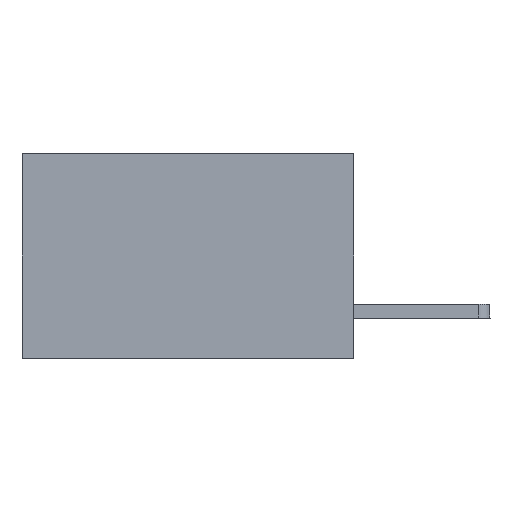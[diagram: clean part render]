
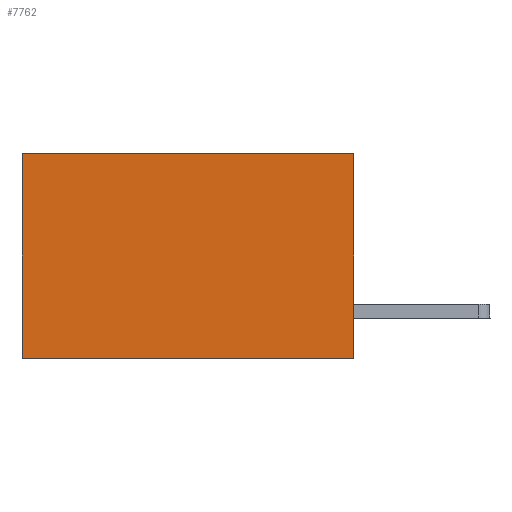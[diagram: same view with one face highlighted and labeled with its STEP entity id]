
A CAD part, left-side view. The second image highlights one B-rep face of the part: STEP entity #7762.
In plain terms, the highlighted planar face has unit normal (-1, 0, 0).
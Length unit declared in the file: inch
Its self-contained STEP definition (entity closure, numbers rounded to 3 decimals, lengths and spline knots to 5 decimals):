
#231 = VERTEX_POINT ( 'NONE', #5318 ) ;
#266 = CARTESIAN_POINT ( 'NONE',  ( 0.2875, 0.6, 0. ) ) ;
#314 = DIRECTION ( 'NONE',  ( 0., 0., -1. ) ) ;
#637 = ORIENTED_EDGE ( 'NONE', *, *, #11480, .T. ) ;
#988 = CARTESIAN_POINT ( 'NONE',  ( 0.2875, 0., 0. ) ) ;
#1458 = CARTESIAN_POINT ( 'NONE',  ( 0.2875, 0., 0. ) ) ;
#1547 = FACE_OUTER_BOUND ( 'NONE', #9340, .T. ) ;
#2187 = LINE ( 'NONE', #3910, #12727 ) ;
#2252 = CARTESIAN_POINT ( 'NONE',  ( 0.2875, 0., -0.37 ) ) ;
#2269 = ORIENTED_EDGE ( 'NONE', *, *, #9729, .T. ) ;
#2368 = DIRECTION ( 'NONE',  ( 0., 1., 0. ) ) ;
#3910 = CARTESIAN_POINT ( 'NONE',  ( 0.2875, 0., 0. ) ) ;
#3998 = VECTOR ( 'NONE', #6832, 39.37008 ) ;
#4287 = VERTEX_POINT ( 'NONE', #12548 ) ;
#4933 = DIRECTION ( 'NONE',  ( 0., 0., -1. ) ) ;
#5099 = EDGE_CURVE ( 'NONE', #5655, #4287, #7421, .T. ) ;
#5167 = EDGE_CURVE ( 'NONE', #4287, #12468, #11554, .T. ) ;
#5318 = CARTESIAN_POINT ( 'NONE',  ( 0.2875, 0.6, 0. ) ) ;
#5651 = ORIENTED_EDGE ( 'NONE', *, *, #5167, .F. ) ;
#5655 = VERTEX_POINT ( 'NONE', #988 ) ;
#6020 = VECTOR ( 'NONE', #314, 39.37008 ) ;
#6258 = CARTESIAN_POINT ( 'NONE',  ( 0.2875, 0., 0. ) ) ;
#6832 = DIRECTION ( 'NONE',  ( 0., 0., -1. ) ) ;
#7421 = LINE ( 'NONE', #6258, #3998 ) ;
#7762 = ADVANCED_FACE ( 'NONE', ( #1547 ), #10022, .F. ) ;
#8261 = CARTESIAN_POINT ( 'NONE',  ( 0.2875, 0.6, -0.37 ) ) ;
#8296 = ORIENTED_EDGE ( 'NONE', *, *, #5099, .F. ) ;
#8690 = LINE ( 'NONE', #266, #6020 ) ;
#9340 = EDGE_LOOP ( 'NONE', ( #2269, #5651, #8296, #637 ) ) ;
#9467 = AXIS2_PLACEMENT_3D ( 'NONE', #1458, #11020, #4933 ) ;
#9729 = EDGE_CURVE ( 'NONE', #231, #12468, #8690, .T. ) ;
#10022 = PLANE ( 'NONE',  #9467 ) ;
#11020 = DIRECTION ( 'NONE',  ( 1., 0., 0. ) ) ;
#11480 = EDGE_CURVE ( 'NONE', #5655, #231, #2187, .T. ) ;
#11554 = LINE ( 'NONE', #2252, #13237 ) ;
#12468 = VERTEX_POINT ( 'NONE', #8261 ) ;
#12548 = CARTESIAN_POINT ( 'NONE',  ( 0.2875, 0., -0.37 ) ) ;
#12727 = VECTOR ( 'NONE', #12863, 39.37008 ) ;
#12863 = DIRECTION ( 'NONE',  ( 0., 1., 0. ) ) ;
#13237 = VECTOR ( 'NONE', #2368, 39.37008 ) ;
